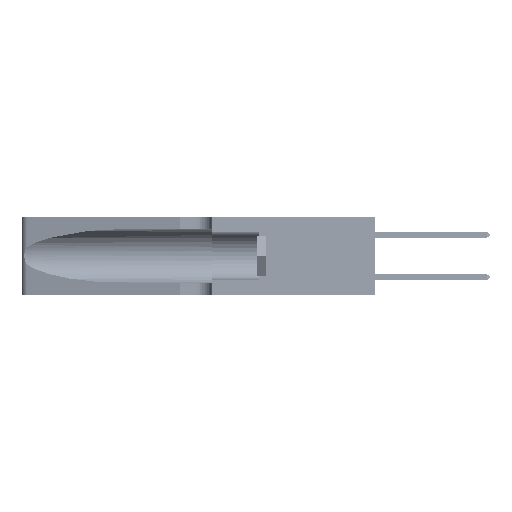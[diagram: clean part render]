
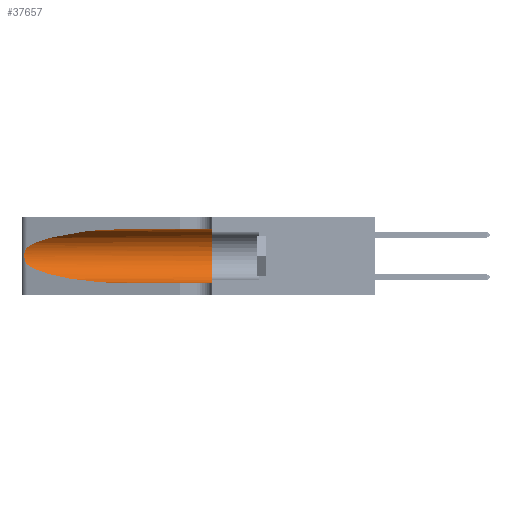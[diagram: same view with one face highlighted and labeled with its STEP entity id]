
A CAD part, left-side view. The second image highlights one B-rep face of the part: STEP entity #37657.
In plain terms, the highlighted cylindrical face has radius 3.308 mm (diameter 6.617 mm), a partial arc.
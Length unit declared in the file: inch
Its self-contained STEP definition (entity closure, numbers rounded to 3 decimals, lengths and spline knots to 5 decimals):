
#261 = CIRCLE ( 'NONE', #5352, 0.13025 ) ;
#673 = CARTESIAN_POINT ( 'NONE',  ( 0.25555, 1.22993, 0.14849 ) ) ;
#2265 = LINE ( 'NONE', #25979, #37811 ) ;
#3694 = CARTESIAN_POINT ( 'NONE',  ( 0.25487, 1.22718, 0.22369 ) ) ;
#4985 = CARTESIAN_POINT ( 'NONE',  ( 0.25487, 1.22718, 0.22369 ) ) ;
#5352 = AXIS2_PLACEMENT_3D ( 'NONE', #23177, #30591, #49445 ) ;
#6562 = ORIENTED_EDGE ( 'NONE', *, *, #36922, .F. ) ;
#7981 = VERTEX_POINT ( 'NONE', #13780 ) ;
#8179 = DIRECTION ( 'NONE',  ( 0., -1., 0. ) ) ;
#8512 = CARTESIAN_POINT ( 'NONE',  ( 0.1305, 1.61858, 0.05475 ) ) ;
#8935 = VERTEX_POINT ( 'NONE', #4985 ) ;
#9960 = VERTEX_POINT ( 'NONE', #29667 ) ;
#11828 = ORIENTED_EDGE ( 'NONE', *, *, #36897, .T. ) ;
#12397 = CARTESIAN_POINT ( 'NONE',  ( 0.25856, 1.23593, 0.16098 ) ) ;
#12717 = FACE_OUTER_BOUND ( 'NONE', #26567, .T. ) ;
#13441 = CARTESIAN_POINT ( 'NONE',  ( 0.1305, 0.35, 0.05475 ) ) ;
#13780 = CARTESIAN_POINT ( 'NONE',  ( 0.1305, 0.35, 0.31525 ) ) ;
#15371 = CARTESIAN_POINT ( 'NONE',  ( 0.25854, 1.2359, 0.20912 ) ) ;
#16026 = CARTESIAN_POINT ( 'NONE',  ( 0.25555, 1.22994, 0.2215 ) ) ;
#16470 = CARTESIAN_POINT ( 'NONE',  ( 0.1305, 0.72297, 0.05475 ) ) ;
#16536 = CARTESIAN_POINT ( 'NONE',  ( 0.26017, 1.23833, 0.17102 ) ) ;
#18598 = DIRECTION ( 'NONE',  ( 0., 0., -1. ) ) ;
#18873 = CARTESIAN_POINT ( 'NONE',  ( 0.25487, 1.22718, 0.14631 ) ) ;
#18942 = EDGE_CURVE ( 'NONE', #42846, #9960, #20320, .T. ) ;
#20320 =( BOUNDED_CURVE ( )  B_SPLINE_CURVE ( 3, ( #24126, #24299, #44319, #16470 ),
 .UNSPECIFIED., .F., .F. ) 
 B_SPLINE_CURVE_WITH_KNOTS ( ( 4, 4 ),
 ( 3.44316, 4.71239 ),
 .UNSPECIFIED. ) 
 CURVE ( )  GEOMETRIC_REPRESENTATION_ITEM ( )  RATIONAL_B_SPLINE_CURVE ( ( 1., 0.87, 0.87, 1. ) ) 
 REPRESENTATION_ITEM ( '' )  );
#20531 = CARTESIAN_POINT ( 'NONE',  ( 0.25639, 1.23186, 0.15144 ) ) ;
#20776 = CYLINDRICAL_SURFACE ( 'NONE', #37384, 0.13025 ) ;
#21929 = CARTESIAN_POINT ( 'NONE',  ( 0.1305, 1.61858, 0.185 ) ) ;
#22529 = ORIENTED_EDGE ( 'NONE', *, *, #41483, .F. ) ;
#23177 = CARTESIAN_POINT ( 'NONE',  ( 0.1305, 0.35, 0.185 ) ) ;
#23540 = CARTESIAN_POINT ( 'NONE',  ( 0.26018, 1.23835, 0.19895 ) ) ;
#23978 = LINE ( 'NONE', #8512, #41409 ) ;
#24033 = CARTESIAN_POINT ( 'NONE',  ( 0.25787, 1.23484, 0.2124 ) ) ;
#24126 = CARTESIAN_POINT ( 'NONE',  ( 0.25487, 1.22718, 0.14631 ) ) ;
#24299 = CARTESIAN_POINT ( 'NONE',  ( 0.2373, 1.15595, 0.08982 ) ) ;
#24856 = EDGE_CURVE ( 'NONE', #8935, #42846, #38233, .T. ) ;
#24892 = CARTESIAN_POINT ( 'NONE',  ( 0.26075, 1.23896, 0.178 ) ) ;
#25979 = CARTESIAN_POINT ( 'NONE',  ( 0.1305, 1.61858, 0.31525 ) ) ;
#26567 = EDGE_LOOP ( 'NONE', ( #45918, #43334, #35814, #11828, #6562, #22529 ) ) ;
#29667 = CARTESIAN_POINT ( 'NONE',  ( 0.1305, 0.72297, 0.05475 ) ) ;
#30195 = CARTESIAN_POINT ( 'NONE',  ( 0.1305, 0.72297, 0.31525 ) ) ;
#30437 = DIRECTION ( 'NONE',  ( 0., -1., 0. ) ) ;
#30591 = DIRECTION ( 'NONE',  ( 0., 1., 0. ) ) ;
#30976 = CARTESIAN_POINT ( 'NONE',  ( 0.2373, 1.15595, 0.28018 ) ) ;
#35125 = VERTEX_POINT ( 'NONE', #30195 ) ;
#35500 = CARTESIAN_POINT ( 'NONE',  ( 0.25487, 1.22718, 0.22369 ) ) ;
#35814 = ORIENTED_EDGE ( 'NONE', *, *, #18942, .T. ) ;
#36402 = CARTESIAN_POINT ( 'NONE',  ( 0.25789, 1.23486, 0.15765 ) ) ;
#36897 = EDGE_CURVE ( 'NONE', #9960, #50206, #23978, .T. ) ;
#36922 = EDGE_CURVE ( 'NONE', #7981, #50206, #261, .T. ) ;
#37384 = AXIS2_PLACEMENT_3D ( 'NONE', #21929, #30437, #18598 ) ;
#37657 = ADVANCED_FACE ( 'NONE', ( #12717 ), #20776, .F. ) ;
#37811 = VECTOR ( 'NONE', #46311, 39.37008 ) ;
#38233 = B_SPLINE_CURVE_WITH_KNOTS ( 'NONE', 3,
 ( #3694, #16026, #43355, #24033, #15371, #23540, #39546, #24892, #16536, #12397, #36402, #20531, #673, #44381 ),
 .UNSPECIFIED., .F., .F.,
 ( 4, 2, 2, 2, 2, 2, 4 ),
 ( 0., 0.00027, 0.00053, 0.00107, 0.0016, 0.00187, 0.00214 ),
 .UNSPECIFIED. ) ;
#39168 = CARTESIAN_POINT ( 'NONE',  ( 0.1305, 0.72297, 0.31525 ) ) ;
#39546 = CARTESIAN_POINT ( 'NONE',  ( 0.26075, 1.23896, 0.19203 ) ) ;
#41409 = VECTOR ( 'NONE', #8179, 39.37008 ) ;
#41483 = EDGE_CURVE ( 'NONE', #35125, #7981, #2265, .T. ) ;
#42846 = VERTEX_POINT ( 'NONE', #18873 ) ;
#43334 = ORIENTED_EDGE ( 'NONE', *, *, #24856, .T. ) ;
#43355 = CARTESIAN_POINT ( 'NONE',  ( 0.25639, 1.23184, 0.21858 ) ) ;
#44245 =( BOUNDED_CURVE ( )  B_SPLINE_CURVE ( 3, ( #39168, #51455, #30976, #35500 ),
 .UNSPECIFIED., .F., .F. ) 
 B_SPLINE_CURVE_WITH_KNOTS ( ( 4, 4 ),
 ( 1.5708, 2.84003 ),
 .UNSPECIFIED. ) 
 CURVE ( )  GEOMETRIC_REPRESENTATION_ITEM ( )  RATIONAL_B_SPLINE_CURVE ( ( 1., 0.87, 0.87, 1. ) ) 
 REPRESENTATION_ITEM ( '' )  );
#44319 = CARTESIAN_POINT ( 'NONE',  ( 0.18966, 0.96281, 0.05475 ) ) ;
#44381 = CARTESIAN_POINT ( 'NONE',  ( 0.25487, 1.22718, 0.14631 ) ) ;
#45918 = ORIENTED_EDGE ( 'NONE', *, *, #50541, .T. ) ;
#46311 = DIRECTION ( 'NONE',  ( 0., -1., 0. ) ) ;
#49445 = DIRECTION ( 'NONE',  ( 0., 0., 1. ) ) ;
#50206 = VERTEX_POINT ( 'NONE', #13441 ) ;
#50541 = EDGE_CURVE ( 'NONE', #35125, #8935, #44245, .T. ) ;
#51455 = CARTESIAN_POINT ( 'NONE',  ( 0.18966, 0.96281, 0.31525 ) ) ;
